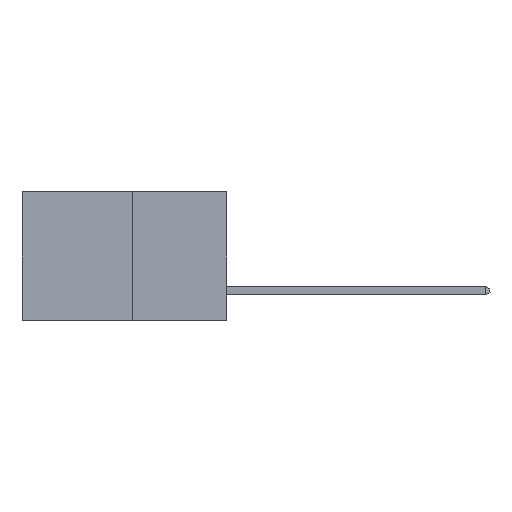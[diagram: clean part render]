
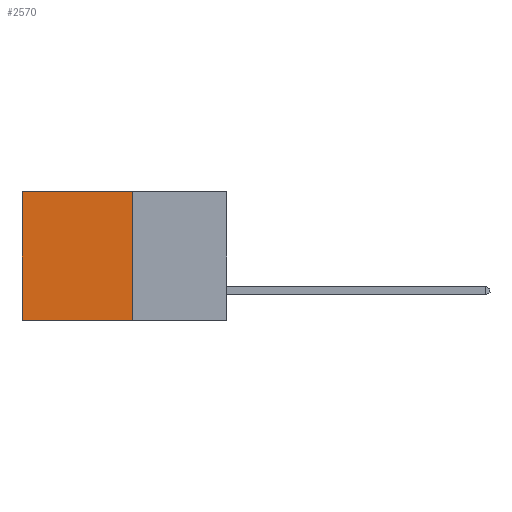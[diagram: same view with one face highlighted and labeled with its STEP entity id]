
A CAD part, left-side view. The second image highlights one B-rep face of the part: STEP entity #2570.
In plain terms, the highlighted planar face has unit normal (-1, 0, 0).
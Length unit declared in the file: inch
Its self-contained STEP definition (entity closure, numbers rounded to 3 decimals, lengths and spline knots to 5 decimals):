
#63 = CARTESIAN_POINT ( 'NONE',  ( 0.277, 0.59, 0. ) ) ;
#126 = VECTOR ( 'NONE', #2315, 39.37008 ) ;
#608 = CARTESIAN_POINT ( 'NONE',  ( 0.277, 0.59, -0.37 ) ) ;
#832 = CARTESIAN_POINT ( 'NONE',  ( 0.277, 0.27, -0.37 ) ) ;
#876 = EDGE_LOOP ( 'NONE', ( #3657, #7369, #8209, #2197 ) ) ;
#1488 = CARTESIAN_POINT ( 'NONE',  ( 0.277, 0.27, 0. ) ) ;
#1595 = PLANE ( 'NONE',  #5703 ) ;
#1626 = DIRECTION ( 'NONE',  ( 0., 0., -1. ) ) ;
#2170 = LINE ( 'NONE', #608, #6410 ) ;
#2178 = CARTESIAN_POINT ( 'NONE',  ( 0.277, 0.27, -0.37 ) ) ;
#2197 = ORIENTED_EDGE ( 'NONE', *, *, #9302, .T. ) ;
#2315 = DIRECTION ( 'NONE',  ( 0., 1., 0. ) ) ;
#2361 = LINE ( 'NONE', #2178, #8397 ) ;
#2474 = EDGE_CURVE ( 'NONE', #6504, #4809, #9004, .T. ) ;
#2570 = ADVANCED_FACE ( 'NONE', ( #8508 ), #1595, .F. ) ;
#2786 = CARTESIAN_POINT ( 'NONE',  ( 0.277, 0.27, -0.37 ) ) ;
#3082 = CARTESIAN_POINT ( 'NONE',  ( 0.277, 0.27, -0.37 ) ) ;
#3657 = ORIENTED_EDGE ( 'NONE', *, *, #8708, .T. ) ;
#4809 = VERTEX_POINT ( 'NONE', #2786 ) ;
#5125 = VECTOR ( 'NONE', #7778, 39.37008 ) ;
#5229 = EDGE_CURVE ( 'NONE', #4809, #7941, #2361, .T. ) ;
#5703 = AXIS2_PLACEMENT_3D ( 'NONE', #832, #6434, #1626 ) ;
#6410 = VECTOR ( 'NONE', #7000, 39.37008 ) ;
#6434 = DIRECTION ( 'NONE',  ( 1., 0., 0. ) ) ;
#6504 = VERTEX_POINT ( 'NONE', #8479 ) ;
#6509 = LINE ( 'NONE', #1488, #126 ) ;
#6758 = DIRECTION ( 'NONE',  ( 0., 1., 0. ) ) ;
#6822 = CARTESIAN_POINT ( 'NONE',  ( 0.277, 0.59, -0.37 ) ) ;
#7000 = DIRECTION ( 'NONE',  ( 0., 0., -1. ) ) ;
#7369 = ORIENTED_EDGE ( 'NONE', *, *, #5229, .F. ) ;
#7778 = DIRECTION ( 'NONE',  ( 0., 0., -1. ) ) ;
#7941 = VERTEX_POINT ( 'NONE', #6822 ) ;
#8209 = ORIENTED_EDGE ( 'NONE', *, *, #2474, .F. ) ;
#8397 = VECTOR ( 'NONE', #6758, 39.37008 ) ;
#8479 = CARTESIAN_POINT ( 'NONE',  ( 0.277, 0.27, 0. ) ) ;
#8508 = FACE_OUTER_BOUND ( 'NONE', #876, .T. ) ;
#8708 = EDGE_CURVE ( 'NONE', #8981, #7941, #2170, .T. ) ;
#8981 = VERTEX_POINT ( 'NONE', #63 ) ;
#9004 = LINE ( 'NONE', #3082, #5125 ) ;
#9302 = EDGE_CURVE ( 'NONE', #6504, #8981, #6509, .T. ) ;
